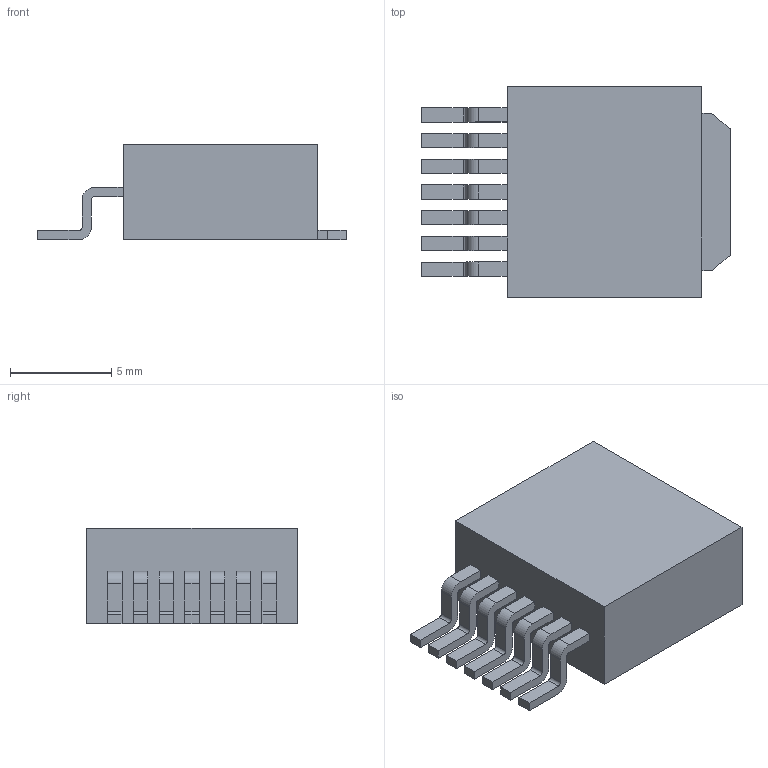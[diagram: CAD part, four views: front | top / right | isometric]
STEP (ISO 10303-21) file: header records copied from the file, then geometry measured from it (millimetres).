
FILE_DESCRIPTION(/* description */ (''),/* implementation_level */ '2;1');
FILE_NAME(/* name */ 'dpak_1583521376508.stp',/* time_stamp */ '2020-03-06T19:03:00+00:00',/* author */ (''),/* organization */ (''),/* preprocessor_version */ 'ST-DEVELOPER v18',/* originating_system */ 'ASM',/* authorisation */ '');
FILE_SCHEMA (('AUTOMOTIVE_DESIGN { 1 0 10303 214 3 1 1 }'));
Length unit declared in the file: millimetre
Products named in the file (1): dpak_1583521376508
Bounding box: 15.25 x 10.4 x 4.7 mm (x, y, z)
Volume: 488.9 mm3; surface area: 507.2 mm2
Topology: 1 solids, 1 shells, 105 faces, 288 edges, 192 vertices
Faces by surface type: plane 77, cylinder 28
Entity records: 3455 total; most frequent: CARTESIAN_POINT 586, ORIENTED_EDGE 576, DIRECTION 556, EDGE_CURVE 288, LINE 232, VECTOR 232, VERTEX_POINT 192, AXIS2_PLACEMENT_3D 162
